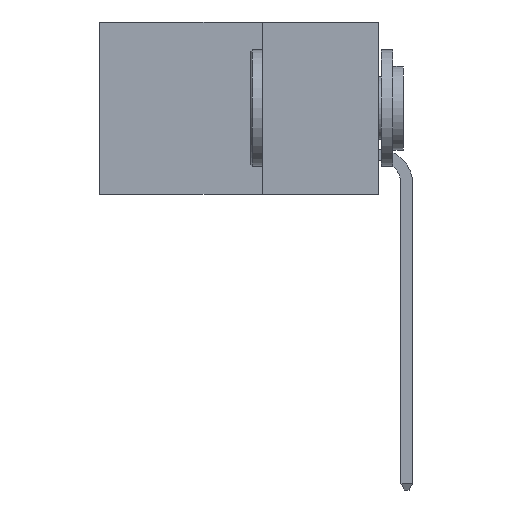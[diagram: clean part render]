
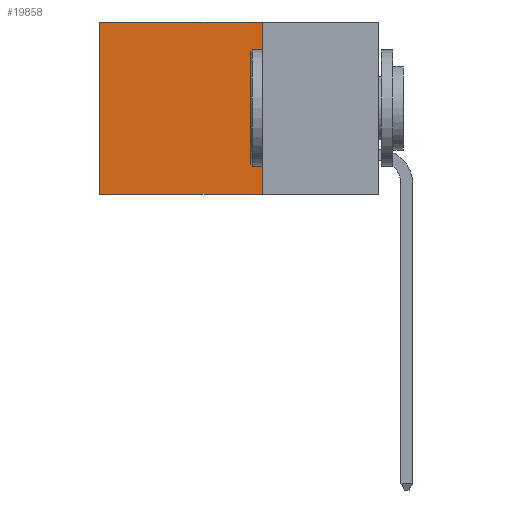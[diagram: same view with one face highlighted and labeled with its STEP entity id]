
A CAD part, left-side view. The second image highlights one B-rep face of the part: STEP entity #19858.
In plain terms, the highlighted planar face has unit normal (-1, 0, 0).
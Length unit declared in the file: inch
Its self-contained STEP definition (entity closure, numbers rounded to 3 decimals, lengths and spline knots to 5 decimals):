
#606 = VECTOR ( 'NONE', #14761, 39.37008 ) ;
#1123 = CARTESIAN_POINT ( 'NONE',  ( 0.2615, 0.6, -0.37 ) ) ;
#1186 = LINE ( 'NONE', #12977, #606 ) ;
#1256 = DIRECTION ( 'NONE',  ( 0., 0., -1. ) ) ;
#3059 = LINE ( 'NONE', #1123, #7368 ) ;
#3137 = DIRECTION ( 'NONE',  ( 0., 0., -1. ) ) ;
#3652 = EDGE_CURVE ( 'NONE', #8904, #15724, #3059, .T. ) ;
#4125 = ORIENTED_EDGE ( 'NONE', *, *, #22830, .F. ) ;
#4577 = CARTESIAN_POINT ( 'NONE',  ( 0.2615, 0.25, -0.37 ) ) ;
#4610 = VERTEX_POINT ( 'NONE', #20498 ) ;
#5929 = ORIENTED_EDGE ( 'NONE', *, *, #3652, .T. ) ;
#5960 = CARTESIAN_POINT ( 'NONE',  ( 0.2615, 0.25, -0.37 ) ) ;
#6899 = EDGE_LOOP ( 'NONE', ( #5929, #4125, #18584, #19238 ) ) ;
#7368 = VECTOR ( 'NONE', #3137, 39.37008 ) ;
#7609 = CARTESIAN_POINT ( 'NONE',  ( 0.2615, 0.6, -0.37 ) ) ;
#7787 = DIRECTION ( 'NONE',  ( 0., 1., 0. ) ) ;
#8904 = VERTEX_POINT ( 'NONE', #20024 ) ;
#9738 = VERTEX_POINT ( 'NONE', #10043 ) ;
#10043 = CARTESIAN_POINT ( 'NONE',  ( 0.2615, 0.25, 0. ) ) ;
#12185 = DIRECTION ( 'NONE',  ( 1., 0., 0. ) ) ;
#12473 = LINE ( 'NONE', #4577, #16803 ) ;
#12977 = CARTESIAN_POINT ( 'NONE',  ( 0.2615, 0.25, 0. ) ) ;
#14122 = FACE_OUTER_BOUND ( 'NONE', #6899, .T. ) ;
#14761 = DIRECTION ( 'NONE',  ( 0., 1., 0. ) ) ;
#15690 = AXIS2_PLACEMENT_3D ( 'NONE', #23042, #12185, #1256 ) ;
#15724 = VERTEX_POINT ( 'NONE', #7609 ) ;
#16803 = VECTOR ( 'NONE', #17500, 39.37008 ) ;
#17500 = DIRECTION ( 'NONE',  ( 0., 0., -1. ) ) ;
#18031 = LINE ( 'NONE', #5960, #18573 ) ;
#18289 = EDGE_CURVE ( 'NONE', #9738, #4610, #12473, .T. ) ;
#18573 = VECTOR ( 'NONE', #7787, 39.37008 ) ;
#18584 = ORIENTED_EDGE ( 'NONE', *, *, #18289, .F. ) ;
#19238 = ORIENTED_EDGE ( 'NONE', *, *, #20670, .T. ) ;
#19858 = ADVANCED_FACE ( 'NONE', ( #14122 ), #21288, .F. ) ;
#20024 = CARTESIAN_POINT ( 'NONE',  ( 0.2615, 0.6, 0. ) ) ;
#20498 = CARTESIAN_POINT ( 'NONE',  ( 0.2615, 0.25, -0.37 ) ) ;
#20670 = EDGE_CURVE ( 'NONE', #9738, #8904, #1186, .T. ) ;
#21288 = PLANE ( 'NONE',  #15690 ) ;
#22830 = EDGE_CURVE ( 'NONE', #4610, #15724, #18031, .T. ) ;
#23042 = CARTESIAN_POINT ( 'NONE',  ( 0.2615, 0.25, -0.37 ) ) ;
